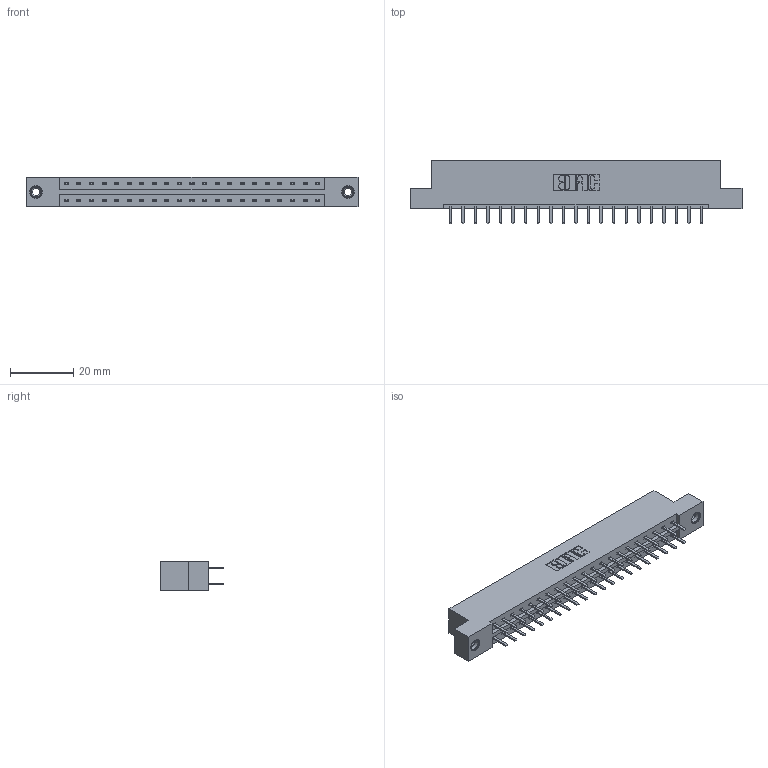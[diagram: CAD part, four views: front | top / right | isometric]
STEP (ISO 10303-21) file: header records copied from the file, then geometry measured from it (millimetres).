
FILE_DESCRIPTION (( 'STEP AP203' ), '1' );
FILE_NAME ('833-042-520-208.STEP', '2020-06-03T20:14:07', ( '' ), ( '' ), 'SwSTEP 2.0', 'SolidWorks 2020', '' );
FILE_SCHEMA (( 'CONFIG_CONTROL_DESIGN' ));
Length unit declared in the file: inch
Products named in the file (4): 345-292-001_345-293-120; 345-250-001_345-250-003-102; 833-042-520-208; 833 Part_Flush - .156 Dia - TI
Assembly tree (45 placements, depth 2):
  833-042-520-208
    833 Part_Flush - .156 Dia - TI
    345-292-001_345-293-120  x42
    345-250-001_345-250-003-102  x2
Bounding box: 104.75 x 20.02 x 9.4 mm (x, y, z)
Volume: 10473 mm3; surface area: 12128.8 mm2
Topology: 45 solids, 45 shells, 2526 faces, 7293 edges, 4742 vertices
Faces by surface type: plane 1698, cylinder 812, cone 12, torus 4
Entity records: 17526 total; most frequent: CARTESIAN_POINT 2925, ORIENTED_EDGE 2842, DIRECTION 2555, EDGE_CURVE 1421, VECTOR 1269, LINE 1269, VERTEX_POINT 940, AXIS2_PLACEMENT_3D 643
